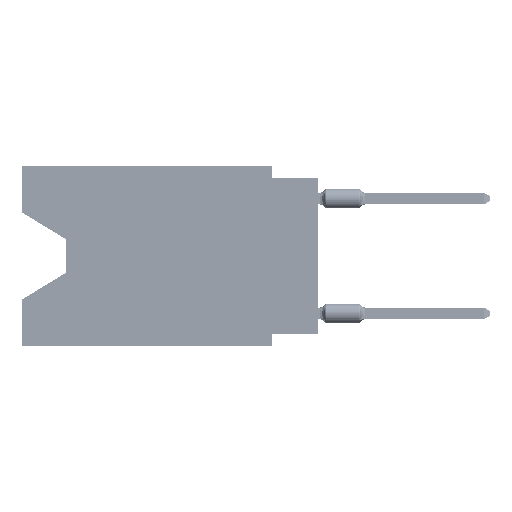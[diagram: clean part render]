
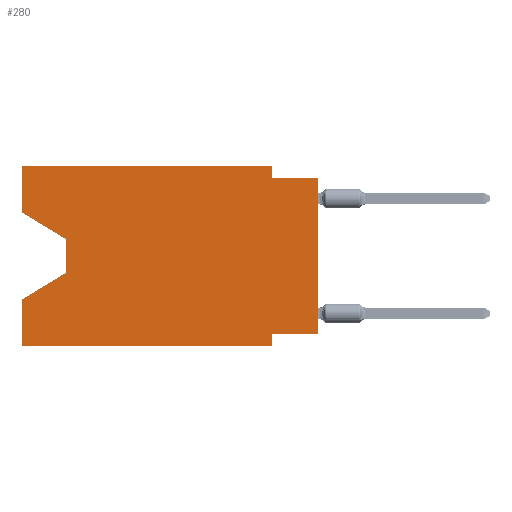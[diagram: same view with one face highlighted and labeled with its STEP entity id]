
A CAD part, left-side view. The second image highlights one B-rep face of the part: STEP entity #280.
In plain terms, the highlighted planar face has unit normal (-1, 0, 0).
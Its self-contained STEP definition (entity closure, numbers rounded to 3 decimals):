
#280 = ADVANCED_FACE ( 'NONE', ( #45918 ), #66791, .F. ) ;
#621 = CARTESIAN_POINT ( 'NONE',  ( 0., 0., -9.271 ) ) ;
#1058 = DIRECTION ( 'NONE',  ( 0., 0., -1. ) ) ;
#2368 = VERTEX_POINT ( 'NONE', #31000 ) ;
#2528 = ORIENTED_EDGE ( 'NONE', *, *, #32099, .F. ) ;
#2593 = VERTEX_POINT ( 'NONE', #55160 ) ;
#2626 = VERTEX_POINT ( 'NONE', #24047 ) ;
#2958 = ORIENTED_EDGE ( 'NONE', *, *, #16012, .T. ) ;
#3027 = CARTESIAN_POINT ( 'NONE',  ( 0., 13.97, -5.893 ) ) ;
#3795 = CARTESIAN_POINT ( 'NONE',  ( 0., 0., -9.271 ) ) ;
#7166 = LINE ( 'NONE', #44452, #50177 ) ;
#7330 = ORIENTED_EDGE ( 'NONE', *, *, #49978, .T. ) ;
#8834 = CARTESIAN_POINT ( 'NONE',  ( 0., 2.54, -9.906 ) ) ;
#8958 = LINE ( 'NONE', #3795, #33322 ) ;
#9570 = VECTOR ( 'NONE', #10491, 1000. ) ;
#9662 = VECTOR ( 'NONE', #39624, 1000. ) ;
#10250 = DIRECTION ( 'NONE',  ( 0., 0.855, -0.519 ) ) ;
#10296 = DIRECTION ( 'NONE',  ( 0., -1., 0. ) ) ;
#10442 = VERTEX_POINT ( 'NONE', #59465 ) ;
#10491 = DIRECTION ( 'NONE',  ( 0., 0., 1. ) ) ;
#10630 = DIRECTION ( 'NONE',  ( 0., -1., 0. ) ) ;
#10634 = LINE ( 'NONE', #32520, #18503 ) ;
#10681 = CARTESIAN_POINT ( 'NONE',  ( 0., 13.97, -4.013 ) ) ;
#11261 = EDGE_CURVE ( 'NONE', #2368, #33776, #53520, .T. ) ;
#11537 = CARTESIAN_POINT ( 'NONE',  ( 0., 2.54, 0. ) ) ;
#12188 = AXIS2_PLACEMENT_3D ( 'NONE', #62642, #57511, #1058 ) ;
#13273 = ORIENTED_EDGE ( 'NONE', *, *, #11261, .F. ) ;
#14095 = DIRECTION ( 'NONE',  ( 0., 1., 0. ) ) ;
#16012 = EDGE_CURVE ( 'NONE', #65391, #33776, #16730, .T. ) ;
#16730 = LINE ( 'NONE', #57127, #43421 ) ;
#17004 = ORIENTED_EDGE ( 'NONE', *, *, #66493, .F. ) ;
#18503 = VECTOR ( 'NONE', #10296, 1000. ) ;
#19136 = LINE ( 'NONE', #39002, #44550 ) ;
#19535 = VERTEX_POINT ( 'NONE', #10681 ) ;
#21538 = ORIENTED_EDGE ( 'NONE', *, *, #41095, .F. ) ;
#21733 = CARTESIAN_POINT ( 'NONE',  ( 0., 13.97, -4.013 ) ) ;
#22690 = DIRECTION ( 'NONE',  ( 0., 0., 1. ) ) ;
#22799 = DIRECTION ( 'NONE',  ( 0., 0., -1. ) ) ;
#24047 = CARTESIAN_POINT ( 'NONE',  ( 0., 0., -0.635 ) ) ;
#27619 = LINE ( 'NONE', #58414, #46415 ) ;
#30235 = VERTEX_POINT ( 'NONE', #61158 ) ;
#30324 = EDGE_CURVE ( 'NONE', #42789, #2626, #31719, .T. ) ;
#30811 = ORIENTED_EDGE ( 'NONE', *, *, #31426, .F. ) ;
#31000 = CARTESIAN_POINT ( 'NONE',  ( 0., 16.383, -9.906 ) ) ;
#31426 = EDGE_CURVE ( 'NONE', #66018, #30235, #38606, .T. ) ;
#31719 = LINE ( 'NONE', #67644, #9570 ) ;
#31969 = VERTEX_POINT ( 'NONE', #55833 ) ;
#32099 = EDGE_CURVE ( 'NONE', #10442, #2626, #10634, .T. ) ;
#32335 = LINE ( 'NONE', #21733, #65197 ) ;
#32520 = CARTESIAN_POINT ( 'NONE',  ( 0., 0., -0.635 ) ) ;
#32985 = CARTESIAN_POINT ( 'NONE',  ( 0., 16.383, 0. ) ) ;
#33137 = ORIENTED_EDGE ( 'NONE', *, *, #30324, .T. ) ;
#33322 = VECTOR ( 'NONE', #14095, 1000. ) ;
#33776 = VERTEX_POINT ( 'NONE', #53970 ) ;
#36891 = EDGE_CURVE ( 'NONE', #19535, #65391, #32335, .T. ) ;
#37241 = ORIENTED_EDGE ( 'NONE', *, *, #36891, .T. ) ;
#37915 = EDGE_CURVE ( 'NONE', #49155, #19535, #19136, .T. ) ;
#38606 = LINE ( 'NONE', #8834, #9662 ) ;
#38791 = ORIENTED_EDGE ( 'NONE', *, *, #52288, .F. ) ;
#39002 = CARTESIAN_POINT ( 'NONE',  ( 0., 16.383, -2.546 ) ) ;
#39624 = DIRECTION ( 'NONE',  ( 0., 0., -1. ) ) ;
#41095 = EDGE_CURVE ( 'NONE', #42789, #66018, #8958, .T. ) ;
#41777 = ORIENTED_EDGE ( 'NONE', *, *, #59462, .F. ) ;
#41932 = EDGE_LOOP ( 'NONE', ( #55738, #37241, #2958, #13273, #7330, #30811, #21538, #33137, #2528, #38791, #17004, #41777 ) ) ;
#42789 = VERTEX_POINT ( 'NONE', #621 ) ;
#43421 = VECTOR ( 'NONE', #10250, 1000. ) ;
#43578 = VECTOR ( 'NONE', #22690, 1000. ) ;
#44452 = CARTESIAN_POINT ( 'NONE',  ( 0., 16.383, 0. ) ) ;
#44550 = VECTOR ( 'NONE', #49943, 1000. ) ;
#44735 = VECTOR ( 'NONE', #10630, 1000. ) ;
#45918 = FACE_OUTER_BOUND ( 'NONE', #41932, .T. ) ;
#46415 = VECTOR ( 'NONE', #52944, 1000. ) ;
#47558 = LINE ( 'NONE', #48249, #44735 ) ;
#48052 = VECTOR ( 'NONE', #22799, 1000. ) ;
#48249 = CARTESIAN_POINT ( 'NONE',  ( 0., 16.383, -9.906 ) ) ;
#49155 = VERTEX_POINT ( 'NONE', #63797 ) ;
#49943 = DIRECTION ( 'NONE',  ( 0., -0.855, -0.519 ) ) ;
#49978 = EDGE_CURVE ( 'NONE', #2368, #30235, #47558, .T. ) ;
#50177 = VECTOR ( 'NONE', #54024, 1000. ) ;
#52288 = EDGE_CURVE ( 'NONE', #31969, #10442, #64563, .T. ) ;
#52944 = DIRECTION ( 'NONE',  ( 0., 0., 1. ) ) ;
#53189 = CARTESIAN_POINT ( 'NONE',  ( 0., 2.54, -9.271 ) ) ;
#53205 = DIRECTION ( 'NONE',  ( 0., 0., -1. ) ) ;
#53520 = LINE ( 'NONE', #32985, #43578 ) ;
#53970 = CARTESIAN_POINT ( 'NONE',  ( 0., 16.383, -7.36 ) ) ;
#54024 = DIRECTION ( 'NONE',  ( 0., -1., 0. ) ) ;
#55160 = CARTESIAN_POINT ( 'NONE',  ( 0., 16.383, 0. ) ) ;
#55738 = ORIENTED_EDGE ( 'NONE', *, *, #37915, .T. ) ;
#55833 = CARTESIAN_POINT ( 'NONE',  ( 0., 2.54, 0. ) ) ;
#57127 = CARTESIAN_POINT ( 'NONE',  ( 0., 13.97, -5.893 ) ) ;
#57511 = DIRECTION ( 'NONE',  ( 1., 0., 0. ) ) ;
#58414 = CARTESIAN_POINT ( 'NONE',  ( 0., 16.383, 0. ) ) ;
#59462 = EDGE_CURVE ( 'NONE', #49155, #2593, #27619, .T. ) ;
#59465 = CARTESIAN_POINT ( 'NONE',  ( 0., 2.54, -0.635 ) ) ;
#61158 = CARTESIAN_POINT ( 'NONE',  ( 0., 2.54, -9.906 ) ) ;
#62642 = CARTESIAN_POINT ( 'NONE',  ( 0., 16.383, 0. ) ) ;
#63797 = CARTESIAN_POINT ( 'NONE',  ( 0., 16.383, -2.546 ) ) ;
#64563 = LINE ( 'NONE', #11537, #48052 ) ;
#65197 = VECTOR ( 'NONE', #53205, 1000. ) ;
#65391 = VERTEX_POINT ( 'NONE', #3027 ) ;
#66018 = VERTEX_POINT ( 'NONE', #53189 ) ;
#66493 = EDGE_CURVE ( 'NONE', #2593, #31969, #7166, .T. ) ;
#66791 = PLANE ( 'NONE',  #12188 ) ;
#67644 = CARTESIAN_POINT ( 'NONE',  ( 0., 0., 0. ) ) ;
